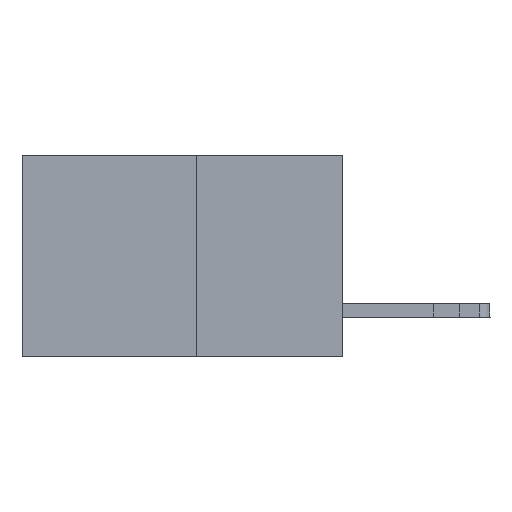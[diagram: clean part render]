
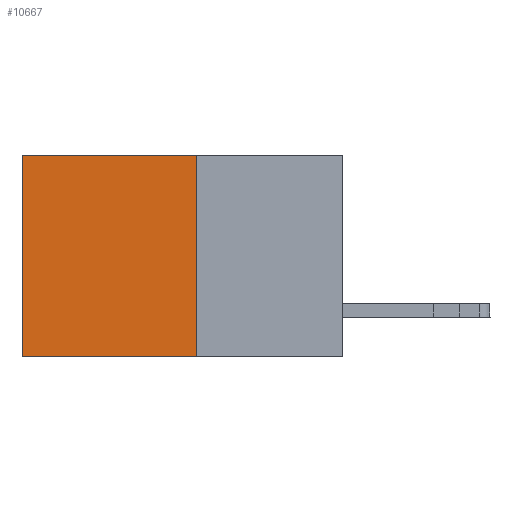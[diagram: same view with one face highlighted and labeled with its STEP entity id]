
A CAD part, left-side view. The second image highlights one B-rep face of the part: STEP entity #10667.
In plain terms, the highlighted planar face has unit normal (-1, 0, 0).
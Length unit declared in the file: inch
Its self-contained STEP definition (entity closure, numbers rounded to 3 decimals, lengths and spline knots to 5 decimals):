
#1671 = EDGE_CURVE ( 'NONE', #21884, #23935, #11083, .T. ) ;
#2945 = LINE ( 'NONE', #22535, #20054 ) ;
#4103 = PLANE ( 'NONE',  #6810 ) ;
#4245 = CARTESIAN_POINT ( 'NONE',  ( 0.277, 0.59, -0.37 ) ) ;
#5419 = CARTESIAN_POINT ( 'NONE',  ( 0.277, 0.27, 0. ) ) ;
#5732 = VECTOR ( 'NONE', #21841, 39.37008 ) ;
#6810 = AXIS2_PLACEMENT_3D ( 'NONE', #21434, #11820, #21053 ) ;
#10667 = ADVANCED_FACE ( 'NONE', ( #13722 ), #4103, .F. ) ;
#11083 = LINE ( 'NONE', #19174, #24457 ) ;
#11633 = VECTOR ( 'NONE', #14697, 39.37008 ) ;
#11820 = DIRECTION ( 'NONE',  ( 1., 0., 0. ) ) ;
#12165 = LINE ( 'NONE', #19885, #11633 ) ;
#13722 = FACE_OUTER_BOUND ( 'NONE', #17035, .T. ) ;
#13938 = VERTEX_POINT ( 'NONE', #20105 ) ;
#14697 = DIRECTION ( 'NONE',  ( 0., 0., -1. ) ) ;
#14791 = VERTEX_POINT ( 'NONE', #24058 ) ;
#15120 = EDGE_CURVE ( 'NONE', #14791, #13938, #2945, .T. ) ;
#15893 = LINE ( 'NONE', #4245, #5732 ) ;
#16739 = EDGE_CURVE ( 'NONE', #21884, #14791, #12165, .T. ) ;
#17035 = EDGE_LOOP ( 'NONE', ( #17380, #21891, #18690, #21382 ) ) ;
#17380 = ORIENTED_EDGE ( 'NONE', *, *, #20782, .T. ) ;
#18690 = ORIENTED_EDGE ( 'NONE', *, *, #16739, .F. ) ;
#19174 = CARTESIAN_POINT ( 'NONE',  ( 0.277, 0.27, 0. ) ) ;
#19885 = CARTESIAN_POINT ( 'NONE',  ( 0.277, 0.27, -0.37 ) ) ;
#20054 = VECTOR ( 'NONE', #24431, 39.37008 ) ;
#20105 = CARTESIAN_POINT ( 'NONE',  ( 0.277, 0.59, -0.37 ) ) ;
#20782 = EDGE_CURVE ( 'NONE', #23935, #13938, #15893, .T. ) ;
#20815 = DIRECTION ( 'NONE',  ( 0., 1., 0. ) ) ;
#21053 = DIRECTION ( 'NONE',  ( 0., 0., -1. ) ) ;
#21382 = ORIENTED_EDGE ( 'NONE', *, *, #1671, .T. ) ;
#21434 = CARTESIAN_POINT ( 'NONE',  ( 0.277, 0.27, -0.37 ) ) ;
#21841 = DIRECTION ( 'NONE',  ( 0., 0., -1. ) ) ;
#21884 = VERTEX_POINT ( 'NONE', #5419 ) ;
#21891 = ORIENTED_EDGE ( 'NONE', *, *, #15120, .F. ) ;
#22535 = CARTESIAN_POINT ( 'NONE',  ( 0.277, 0.27, -0.37 ) ) ;
#23068 = CARTESIAN_POINT ( 'NONE',  ( 0.277, 0.59, 0. ) ) ;
#23935 = VERTEX_POINT ( 'NONE', #23068 ) ;
#24058 = CARTESIAN_POINT ( 'NONE',  ( 0.277, 0.27, -0.37 ) ) ;
#24431 = DIRECTION ( 'NONE',  ( 0., 1., 0. ) ) ;
#24457 = VECTOR ( 'NONE', #20815, 39.37008 ) ;
